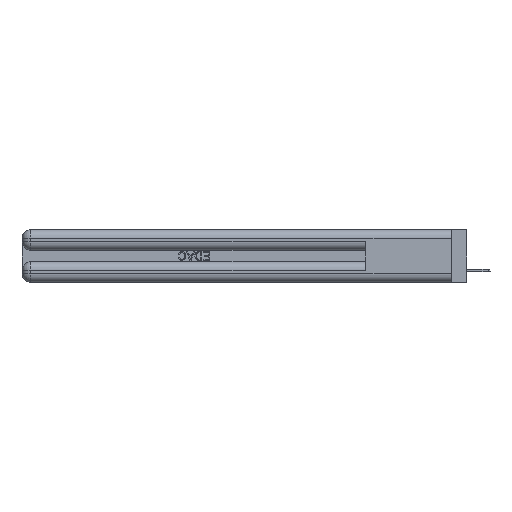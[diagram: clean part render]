
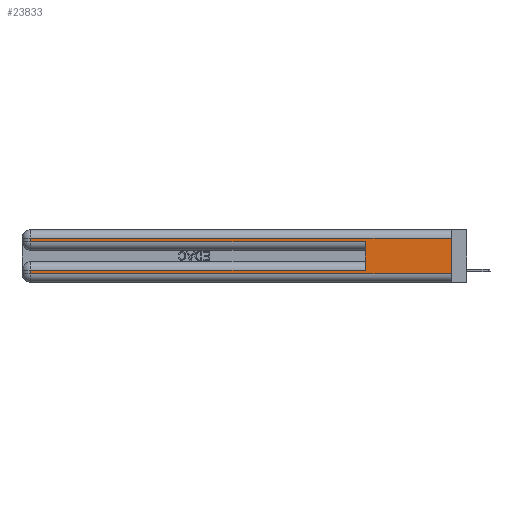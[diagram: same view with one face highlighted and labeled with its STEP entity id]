
A CAD part, left-side view. The second image highlights one B-rep face of the part: STEP entity #23833.
In plain terms, the highlighted planar face has unit normal (-1, 0, 0).
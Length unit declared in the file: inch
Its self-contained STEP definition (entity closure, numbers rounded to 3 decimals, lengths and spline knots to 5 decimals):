
#119 = CARTESIAN_POINT ( 'NONE',  ( 0., 2.94, 0.37 ) ) ;
#1092 = LINE ( 'NONE', #9474, #32301 ) ;
#1325 = CARTESIAN_POINT ( 'NONE',  ( 0., 0., 0.285 ) ) ;
#1748 = DIRECTION ( 'NONE',  ( 1., 0., 0. ) ) ;
#1980 = CARTESIAN_POINT ( 'NONE',  ( 0., 0., 0.06 ) ) ;
#2670 = ORIENTED_EDGE ( 'NONE', *, *, #17535, .T. ) ;
#2828 = EDGE_CURVE ( 'NONE', #23869, #24163, #1092, .T. ) ;
#2902 = ORIENTED_EDGE ( 'NONE', *, *, #42081, .T. ) ;
#4254 = ORIENTED_EDGE ( 'NONE', *, *, #6341, .T. ) ;
#4650 = EDGE_CURVE ( 'NONE', #35755, #36864, #44014, .T. ) ;
#4815 = LINE ( 'NONE', #1325, #42213 ) ;
#4978 = DIRECTION ( 'NONE',  ( 0., -1., 0. ) ) ;
#6341 = EDGE_CURVE ( 'NONE', #22223, #9085, #9947, .T. ) ;
#9058 = DIRECTION ( 'NONE',  ( 0., 0., -1. ) ) ;
#9085 = VERTEX_POINT ( 'NONE', #45483 ) ;
#9153 = ORIENTED_EDGE ( 'NONE', *, *, #40486, .T. ) ;
#9474 = CARTESIAN_POINT ( 'NONE',  ( 0., 0., 0.31 ) ) ;
#9947 = LINE ( 'NONE', #1980, #20731 ) ;
#10878 = ORIENTED_EDGE ( 'NONE', *, *, #19825, .T. ) ;
#11863 = DIRECTION ( 'NONE',  ( 0., 1., 0. ) ) ;
#12306 = ORIENTED_EDGE ( 'NONE', *, *, #4650, .F. ) ;
#12494 = CARTESIAN_POINT ( 'NONE',  ( 0., 0., 0.37 ) ) ;
#13178 = VECTOR ( 'NONE', #14942, 39.37008 ) ;
#13252 = CARTESIAN_POINT ( 'NONE',  ( 0., 2.94, 0.285 ) ) ;
#14409 = CARTESIAN_POINT ( 'NONE',  ( 0., 0.6, 0.145 ) ) ;
#14942 = DIRECTION ( 'NONE',  ( 0., 0., -1. ) ) ;
#16146 = LINE ( 'NONE', #12494, #27542 ) ;
#17535 = EDGE_CURVE ( 'NONE', #35755, #45882, #18653, .T. ) ;
#18653 = LINE ( 'NONE', #44948, #35665 ) ;
#19825 = EDGE_CURVE ( 'NONE', #33515, #36864, #4815, .T. ) ;
#20731 = VECTOR ( 'NONE', #45685, 39.37008 ) ;
#22223 = VERTEX_POINT ( 'NONE', #32815 ) ;
#23378 = ORIENTED_EDGE ( 'NONE', *, *, #40468, .F. ) ;
#23708 = VECTOR ( 'NONE', #34096, 39.37008 ) ;
#23833 = ADVANCED_FACE ( 'NONE', ( #26977 ), #26765, .F. ) ;
#23869 = VERTEX_POINT ( 'NONE', #27781 ) ;
#24163 = VERTEX_POINT ( 'NONE', #26380 ) ;
#26380 = CARTESIAN_POINT ( 'NONE',  ( 0., 2.94, 0.31 ) ) ;
#26765 = PLANE ( 'NONE',  #40282 ) ;
#26940 = VECTOR ( 'NONE', #37780, 39.37008 ) ;
#26977 = FACE_OUTER_BOUND ( 'NONE', #29436, .T. ) ;
#27542 = VECTOR ( 'NONE', #34796, 39.37008 ) ;
#27781 = CARTESIAN_POINT ( 'NONE',  ( 0., 0., 0.31 ) ) ;
#29178 = LINE ( 'NONE', #34308, #26940 ) ;
#29436 = EDGE_LOOP ( 'NONE', ( #23378, #41594, #2902, #10878, #12306, #2670, #9153, #4254 ) ) ;
#30714 = CARTESIAN_POINT ( 'NONE',  ( 0., 0., 0.37 ) ) ;
#32301 = VECTOR ( 'NONE', #34764, 39.37008 ) ;
#32815 = CARTESIAN_POINT ( 'NONE',  ( 0., 2.94, 0.06 ) ) ;
#33515 = VERTEX_POINT ( 'NONE', #13252 ) ;
#34096 = DIRECTION ( 'NONE',  ( 0., 0., 1. ) ) ;
#34308 = CARTESIAN_POINT ( 'NONE',  ( 0., 2.94, 0.37 ) ) ;
#34764 = DIRECTION ( 'NONE',  ( 0., 1., 0. ) ) ;
#34796 = DIRECTION ( 'NONE',  ( 0., 0., -1. ) ) ;
#35603 = CARTESIAN_POINT ( 'NONE',  ( 0., 0.6, 0.085 ) ) ;
#35665 = VECTOR ( 'NONE', #11863, 39.37008 ) ;
#35755 = VERTEX_POINT ( 'NONE', #35603 ) ;
#35820 = LINE ( 'NONE', #119, #13178 ) ;
#36864 = VERTEX_POINT ( 'NONE', #45461 ) ;
#37780 = DIRECTION ( 'NONE',  ( 0., 0., -1. ) ) ;
#38455 = CARTESIAN_POINT ( 'NONE',  ( 0., 2.94, 0.085 ) ) ;
#40282 = AXIS2_PLACEMENT_3D ( 'NONE', #30714, #1748, #9058 ) ;
#40468 = EDGE_CURVE ( 'NONE', #23869, #9085, #16146, .T. ) ;
#40486 = EDGE_CURVE ( 'NONE', #45882, #22223, #29178, .T. ) ;
#41594 = ORIENTED_EDGE ( 'NONE', *, *, #2828, .T. ) ;
#42081 = EDGE_CURVE ( 'NONE', #24163, #33515, #35820, .T. ) ;
#42213 = VECTOR ( 'NONE', #4978, 39.37008 ) ;
#44014 = LINE ( 'NONE', #14409, #23708 ) ;
#44948 = CARTESIAN_POINT ( 'NONE',  ( 0., 0., 0.085 ) ) ;
#45461 = CARTESIAN_POINT ( 'NONE',  ( 0., 0.6, 0.285 ) ) ;
#45483 = CARTESIAN_POINT ( 'NONE',  ( 0., 0., 0.06 ) ) ;
#45685 = DIRECTION ( 'NONE',  ( 0., -1., 0. ) ) ;
#45882 = VERTEX_POINT ( 'NONE', #38455 ) ;
